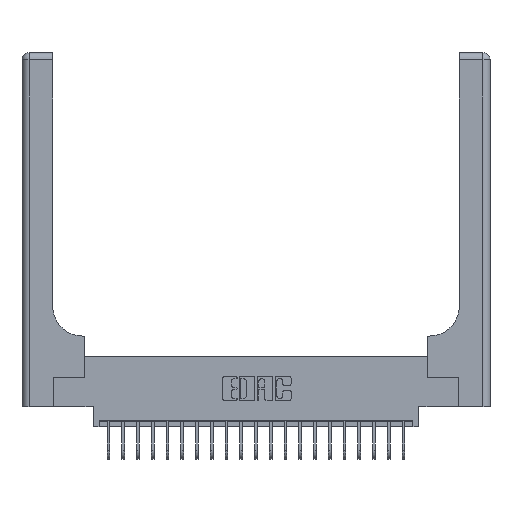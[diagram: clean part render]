
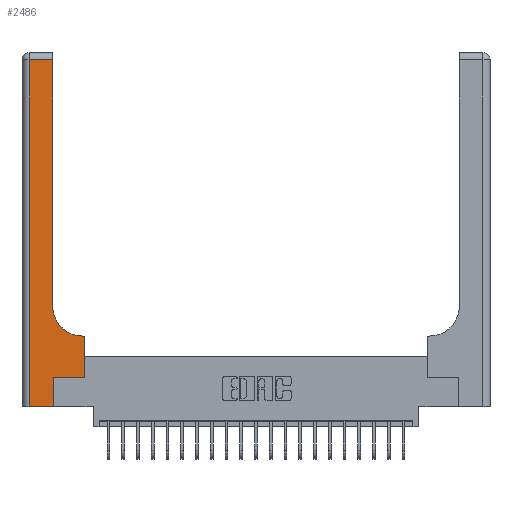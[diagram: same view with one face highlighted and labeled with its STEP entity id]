
A CAD part, top view. The second image highlights one B-rep face of the part: STEP entity #2486.
In plain terms, the highlighted planar face has unit normal (0, 0, 1).
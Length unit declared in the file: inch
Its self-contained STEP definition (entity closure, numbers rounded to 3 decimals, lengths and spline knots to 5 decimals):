
#96 = CARTESIAN_POINT ( 'NONE',  ( 0.265, 0.25, 0.37 ) ) ;
#116 = VERTEX_POINT ( 'NONE', #17563 ) ;
#719 = FACE_OUTER_BOUND ( 'NONE', #13666, .T. ) ;
#991 = AXIS2_PLACEMENT_3D ( 'NONE', #8986, #13921, #20633 ) ;
#1216 = CARTESIAN_POINT ( 'NONE',  ( 0.528, 0.25, 0.37 ) ) ;
#1583 = CARTESIAN_POINT ( 'NONE',  ( 0.26, 3., 0.37 ) ) ;
#1627 = VECTOR ( 'NONE', #17123, 39.37008 ) ;
#1957 = CIRCLE ( 'NONE', #991, 0.25 ) ;
#2381 = LINE ( 'NONE', #13984, #7713 ) ;
#2486 = ADVANCED_FACE ( 'NONE', ( #719 ), #8024, .F. ) ;
#2766 = EDGE_CURVE ( 'NONE', #17726, #20439, #1957, .T. ) ;
#3121 = EDGE_CURVE ( 'NONE', #6722, #17262, #4813, .T. ) ;
#3167 = DIRECTION ( 'NONE',  ( 0., 1., 0. ) ) ;
#3309 = EDGE_CURVE ( 'NONE', #20439, #12529, #6851, .T. ) ;
#3893 = ORIENTED_EDGE ( 'NONE', *, *, #6909, .T. ) ;
#4131 = EDGE_CURVE ( 'NONE', #116, #6722, #2381, .T. ) ;
#4163 = ORIENTED_EDGE ( 'NONE', *, *, #11850, .T. ) ;
#4805 = CARTESIAN_POINT ( 'NONE',  ( 0.06, 2.94, 0.37 ) ) ;
#4813 = LINE ( 'NONE', #11492, #11225 ) ;
#5254 = DIRECTION ( 'NONE',  ( 0., 1., 0. ) ) ;
#5301 = EDGE_CURVE ( 'NONE', #12529, #13619, #12269, .T. ) ;
#5928 = VECTOR ( 'NONE', #19174, 39.37008 ) ;
#6722 = VERTEX_POINT ( 'NONE', #11156 ) ;
#6851 = LINE ( 'NONE', #1583, #7079 ) ;
#6901 = CARTESIAN_POINT ( 'NONE',  ( 0.26, 0.85, 0.37 ) ) ;
#6909 = EDGE_CURVE ( 'NONE', #15526, #17726, #15090, .T. ) ;
#7079 = VECTOR ( 'NONE', #13308, 39.37008 ) ;
#7242 = CARTESIAN_POINT ( 'NONE',  ( 0., 2.94, 0.37 ) ) ;
#7713 = VECTOR ( 'NONE', #20699, 39.37008 ) ;
#8024 = PLANE ( 'NONE',  #12099 ) ;
#8133 = CARTESIAN_POINT ( 'NONE',  ( 0.528, 0.6, 0.37 ) ) ;
#8141 = VECTOR ( 'NONE', #5254, 39.37008 ) ;
#8875 = ORIENTED_EDGE ( 'NONE', *, *, #11307, .T. ) ;
#8986 = CARTESIAN_POINT ( 'NONE',  ( 0.51, 0.85, 0.37 ) ) ;
#9218 = LINE ( 'NONE', #15908, #1627 ) ;
#9831 = CARTESIAN_POINT ( 'NONE',  ( 0.26, 2.94, 0.37 ) ) ;
#10683 = DIRECTION ( 'NONE',  ( -1., 0., 0. ) ) ;
#11156 = CARTESIAN_POINT ( 'NONE',  ( 0.265, 0., 0.37 ) ) ;
#11225 = VECTOR ( 'NONE', #3167, 39.37008 ) ;
#11304 = ORIENTED_EDGE ( 'NONE', *, *, #21307, .T. ) ;
#11307 = EDGE_CURVE ( 'NONE', #13619, #116, #13100, .T. ) ;
#11492 = CARTESIAN_POINT ( 'NONE',  ( 0.265, 0., 0.37 ) ) ;
#11804 = CARTESIAN_POINT ( 'NONE',  ( 0.26, 0.6, 0.37 ) ) ;
#11850 = EDGE_CURVE ( 'NONE', #17262, #20254, #9218, .T. ) ;
#12099 = AXIS2_PLACEMENT_3D ( 'NONE', #12330, #18100, #10683 ) ;
#12269 = LINE ( 'NONE', #7242, #5928 ) ;
#12330 = CARTESIAN_POINT ( 'NONE',  ( 0., 3., 0.37 ) ) ;
#12529 = VERTEX_POINT ( 'NONE', #9831 ) ;
#13100 = LINE ( 'NONE', #17525, #15968 ) ;
#13308 = DIRECTION ( 'NONE',  ( 0., 1., 0. ) ) ;
#13619 = VERTEX_POINT ( 'NONE', #4805 ) ;
#13666 = EDGE_LOOP ( 'NONE', ( #17719, #20626, #8875, #15042, #21603, #4163, #11304, #3893, #19185 ) ) ;
#13921 = DIRECTION ( 'NONE',  ( 0., 0., -1. ) ) ;
#13984 = CARTESIAN_POINT ( 'NONE',  ( 0., 0., 0.37 ) ) ;
#15042 = ORIENTED_EDGE ( 'NONE', *, *, #4131, .T. ) ;
#15090 = LINE ( 'NONE', #11804, #19470 ) ;
#15526 = VERTEX_POINT ( 'NONE', #8133 ) ;
#15872 = DIRECTION ( 'NONE',  ( 0., -1., 0. ) ) ;
#15908 = CARTESIAN_POINT ( 'NONE',  ( 0.265, 0.25, 0.37 ) ) ;
#15968 = VECTOR ( 'NONE', #15872, 39.37008 ) ;
#16743 = DIRECTION ( 'NONE',  ( -1., 0., 0. ) ) ;
#16873 = LINE ( 'NONE', #20291, #8141 ) ;
#17123 = DIRECTION ( 'NONE',  ( 1., 0., 0. ) ) ;
#17262 = VERTEX_POINT ( 'NONE', #96 ) ;
#17525 = CARTESIAN_POINT ( 'NONE',  ( 0.06, 3., 0.37 ) ) ;
#17563 = CARTESIAN_POINT ( 'NONE',  ( 0.06, 0., 0.37 ) ) ;
#17719 = ORIENTED_EDGE ( 'NONE', *, *, #3309, .T. ) ;
#17726 = VERTEX_POINT ( 'NONE', #20587 ) ;
#18100 = DIRECTION ( 'NONE',  ( 0., 0., -1. ) ) ;
#19174 = DIRECTION ( 'NONE',  ( -1., 0., 0. ) ) ;
#19185 = ORIENTED_EDGE ( 'NONE', *, *, #2766, .T. ) ;
#19470 = VECTOR ( 'NONE', #16743, 39.37008 ) ;
#20254 = VERTEX_POINT ( 'NONE', #1216 ) ;
#20291 = CARTESIAN_POINT ( 'NONE',  ( 0.528, 0.25, 0.37 ) ) ;
#20439 = VERTEX_POINT ( 'NONE', #6901 ) ;
#20587 = CARTESIAN_POINT ( 'NONE',  ( 0.51, 0.6, 0.37 ) ) ;
#20626 = ORIENTED_EDGE ( 'NONE', *, *, #5301, .T. ) ;
#20633 = DIRECTION ( 'NONE',  ( 1., 0., 0. ) ) ;
#20699 = DIRECTION ( 'NONE',  ( 1., 0., 0. ) ) ;
#21307 = EDGE_CURVE ( 'NONE', #20254, #15526, #16873, .T. ) ;
#21603 = ORIENTED_EDGE ( 'NONE', *, *, #3121, .T. ) ;
